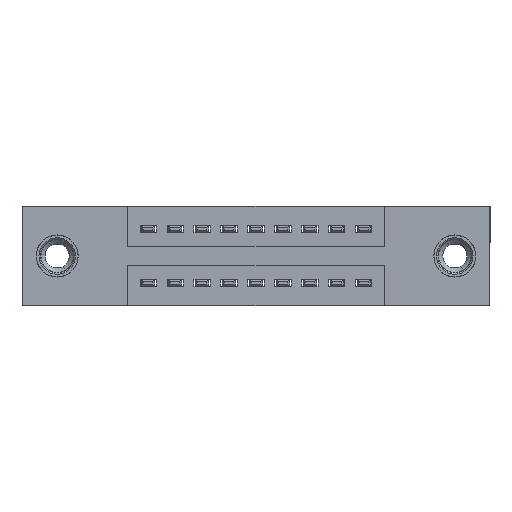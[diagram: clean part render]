
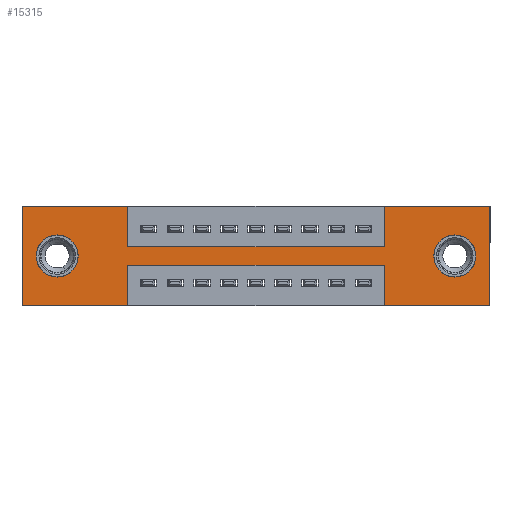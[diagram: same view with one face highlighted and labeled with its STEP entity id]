
A CAD part, front view. The second image highlights one B-rep face of the part: STEP entity #15315.
In plain terms, the highlighted planar face has unit normal (0, -1, 0).
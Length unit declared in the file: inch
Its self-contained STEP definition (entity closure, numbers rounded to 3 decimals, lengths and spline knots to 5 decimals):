
#8 = VECTOR ( 'NONE', #11460, 39.37008 ) ;
#34 = FACE_BOUND ( 'NONE', #10789, .T. ) ;
#126 = CARTESIAN_POINT ( 'NONE',  ( 1.735, 0., -0.37 ) ) ;
#457 = VECTOR ( 'NONE', #1147, 39.37008 ) ;
#826 = CARTESIAN_POINT ( 'NONE',  ( 0.3925, 0., -0.37 ) ) ;
#936 = EDGE_CURVE ( 'NONE', #4161, #10772, #6106, .T. ) ;
#960 = CARTESIAN_POINT ( 'NONE',  ( 0.3925, 0., -0.15 ) ) ;
#1044 = ORIENTED_EDGE ( 'NONE', *, *, #4124, .F. ) ;
#1058 = VERTEX_POINT ( 'NONE', #1745 ) ;
#1147 = DIRECTION ( 'NONE',  ( 0., 0., -1. ) ) ;
#1165 = VERTEX_POINT ( 'NONE', #13339 ) ;
#1525 = CARTESIAN_POINT ( 'NONE',  ( 1.3425, 0., -0.15 ) ) ;
#1726 = VERTEX_POINT ( 'NONE', #2526 ) ;
#1735 = CARTESIAN_POINT ( 'NONE',  ( 1.735, 0., 0. ) ) ;
#1745 = CARTESIAN_POINT ( 'NONE',  ( 0.13, 0., -0.263 ) ) ;
#1762 = AXIS2_PLACEMENT_3D ( 'NONE', #4137, #12771, #5459 ) ;
#1805 = AXIS2_PLACEMENT_3D ( 'NONE', #14011, #6840, #15204 ) ;
#1809 = AXIS2_PLACEMENT_3D ( 'NONE', #8352, #13079, #5833 ) ;
#1891 = CARTESIAN_POINT ( 'NONE',  ( 1.605, 0., -0.185 ) ) ;
#1919 = ORIENTED_EDGE ( 'NONE', *, *, #4104, .F. ) ;
#1977 = CARTESIAN_POINT ( 'NONE',  ( 1.3425, 0., -0.22 ) ) ;
#2094 = ORIENTED_EDGE ( 'NONE', *, *, #14705, .F. ) ;
#2177 = LINE ( 'NONE', #9393, #14913 ) ;
#2216 = LINE ( 'NONE', #7246, #14951 ) ;
#2290 = EDGE_CURVE ( 'NONE', #14207, #11654, #2216, .T. ) ;
#2526 = CARTESIAN_POINT ( 'NONE',  ( 1.3425, 0., 0. ) ) ;
#2630 = CARTESIAN_POINT ( 'NONE',  ( 0.3925, 0., -0.37 ) ) ;
#2646 = ORIENTED_EDGE ( 'NONE', *, *, #936, .F. ) ;
#2746 = FACE_BOUND ( 'NONE', #7208, .T. ) ;
#3183 = DIRECTION ( 'NONE',  ( 0., 0., -1. ) ) ;
#3472 = VERTEX_POINT ( 'NONE', #13127 ) ;
#3543 = ORIENTED_EDGE ( 'NONE', *, *, #13619, .T. ) ;
#3743 = AXIS2_PLACEMENT_3D ( 'NONE', #1891, #10708, #3183 ) ;
#3764 = VECTOR ( 'NONE', #7414, 39.37008 ) ;
#3813 = DIRECTION ( 'NONE',  ( -1., 0., 0. ) ) ;
#4104 = EDGE_CURVE ( 'NONE', #5270, #13709, #4605, .T. ) ;
#4124 = EDGE_CURVE ( 'NONE', #13709, #6918, #4186, .T. ) ;
#4137 = CARTESIAN_POINT ( 'NONE',  ( 1.605, 0., -0.185 ) ) ;
#4161 = VERTEX_POINT ( 'NONE', #13114 ) ;
#4171 = LINE ( 'NONE', #15673, #3764 ) ;
#4186 = LINE ( 'NONE', #14251, #7646 ) ;
#4452 = VERTEX_POINT ( 'NONE', #126 ) ;
#4508 = PLANE ( 'NONE',  #1809 ) ;
#4605 = LINE ( 'NONE', #11854, #13956 ) ;
#4683 = CARTESIAN_POINT ( 'NONE',  ( 0., 0., 0. ) ) ;
#4689 = EDGE_CURVE ( 'NONE', #11654, #5270, #4171, .T. ) ;
#4876 = CARTESIAN_POINT ( 'NONE',  ( 0.3925, 0., -0.22 ) ) ;
#4964 = EDGE_CURVE ( 'NONE', #3472, #14207, #7014, .T. ) ;
#4968 = CIRCLE ( 'NONE', #1762, 0.078 ) ;
#5057 = EDGE_CURVE ( 'NONE', #10867, #1058, #12298, .T. ) ;
#5081 = DIRECTION ( 'NONE',  ( 0., 1., 0. ) ) ;
#5207 = EDGE_CURVE ( 'NONE', #11205, #1726, #7616, .T. ) ;
#5270 = VERTEX_POINT ( 'NONE', #4683 ) ;
#5459 = DIRECTION ( 'NONE',  ( 0., 0., -1. ) ) ;
#5679 = DIRECTION ( 'NONE',  ( 1., 0., 0. ) ) ;
#5729 = CARTESIAN_POINT ( 'NONE',  ( 0.3925, 0., -0.15 ) ) ;
#5833 = DIRECTION ( 'NONE',  ( 0., 0., -1. ) ) ;
#5882 = CARTESIAN_POINT ( 'NONE',  ( 1.3425, 0., 0. ) ) ;
#5897 = LINE ( 'NONE', #4876, #12011 ) ;
#5986 = EDGE_CURVE ( 'NONE', #6918, #11205, #12764, .T. ) ;
#6022 = LINE ( 'NONE', #6444, #14882 ) ;
#6106 = LINE ( 'NONE', #12566, #12930 ) ;
#6213 = ORIENTED_EDGE ( 'NONE', *, *, #15624, .F. ) ;
#6444 = CARTESIAN_POINT ( 'NONE',  ( 0., 0., -0.37 ) ) ;
#6611 = EDGE_CURVE ( 'NONE', #10772, #3472, #5897, .T. ) ;
#6775 = ORIENTED_EDGE ( 'NONE', *, *, #2290, .F. ) ;
#6840 = DIRECTION ( 'NONE',  ( 0., 1., 0. ) ) ;
#6918 = VERTEX_POINT ( 'NONE', #5729 ) ;
#6990 = DIRECTION ( 'NONE',  ( 1., 0., 0. ) ) ;
#7014 = LINE ( 'NONE', #2630, #8 ) ;
#7073 = EDGE_CURVE ( 'NONE', #1058, #10867, #14374, .T. ) ;
#7094 = DIRECTION ( 'NONE',  ( 0., 0., -1. ) ) ;
#7132 = ORIENTED_EDGE ( 'NONE', *, *, #5057, .T. ) ;
#7208 = EDGE_LOOP ( 'NONE', ( #3543, #15861 ) ) ;
#7246 = CARTESIAN_POINT ( 'NONE',  ( 0., 0., -0.37 ) ) ;
#7414 = DIRECTION ( 'NONE',  ( 0., 0., 1. ) ) ;
#7616 = LINE ( 'NONE', #5882, #10794 ) ;
#7646 = VECTOR ( 'NONE', #7094, 39.37008 ) ;
#7765 = VERTEX_POINT ( 'NONE', #8893 ) ;
#7897 = CARTESIAN_POINT ( 'NONE',  ( 0., 0., -0.37 ) ) ;
#8352 = CARTESIAN_POINT ( 'NONE',  ( 0., 0., -0.37 ) ) ;
#8463 = ORIENTED_EDGE ( 'NONE', *, *, #7073, .T. ) ;
#8473 = ORIENTED_EDGE ( 'NONE', *, *, #5986, .F. ) ;
#8501 = CARTESIAN_POINT ( 'NONE',  ( 0.3925, 0., 0. ) ) ;
#8893 = CARTESIAN_POINT ( 'NONE',  ( 1.605, 0., -0.107 ) ) ;
#9007 = CIRCLE ( 'NONE', #3743, 0.078 ) ;
#9393 = CARTESIAN_POINT ( 'NONE',  ( 0., 0., 0. ) ) ;
#9606 = VECTOR ( 'NONE', #13431, 39.37008 ) ;
#9949 = EDGE_CURVE ( 'NONE', #11763, #4452, #10622, .T. ) ;
#10062 = ORIENTED_EDGE ( 'NONE', *, *, #6611, .F. ) ;
#10617 = EDGE_CURVE ( 'NONE', #1165, #7765, #4968, .T. ) ;
#10622 = LINE ( 'NONE', #15905, #457 ) ;
#10664 = ORIENTED_EDGE ( 'NONE', *, *, #5207, .F. ) ;
#10708 = DIRECTION ( 'NONE',  ( 0., 1., 0. ) ) ;
#10772 = VERTEX_POINT ( 'NONE', #1977 ) ;
#10789 = EDGE_LOOP ( 'NONE', ( #7132, #8463 ) ) ;
#10794 = VECTOR ( 'NONE', #11974, 39.37008 ) ;
#10867 = VERTEX_POINT ( 'NONE', #15685 ) ;
#11205 = VERTEX_POINT ( 'NONE', #1525 ) ;
#11275 = ORIENTED_EDGE ( 'NONE', *, *, #4689, .F. ) ;
#11460 = DIRECTION ( 'NONE',  ( 0., 0., -1. ) ) ;
#11654 = VERTEX_POINT ( 'NONE', #7897 ) ;
#11763 = VERTEX_POINT ( 'NONE', #1735 ) ;
#11854 = CARTESIAN_POINT ( 'NONE',  ( 0., 0., 0. ) ) ;
#11974 = DIRECTION ( 'NONE',  ( 0., 0., 1. ) ) ;
#12011 = VECTOR ( 'NONE', #15775, 39.37008 ) ;
#12298 = CIRCLE ( 'NONE', #1805, 0.078 ) ;
#12433 = CARTESIAN_POINT ( 'NONE',  ( 0.13, 0., -0.185 ) ) ;
#12566 = CARTESIAN_POINT ( 'NONE',  ( 1.3425, 0., -0.37 ) ) ;
#12677 = FACE_OUTER_BOUND ( 'NONE', #14859, .T. ) ;
#12764 = LINE ( 'NONE', #960, #9606 ) ;
#12771 = DIRECTION ( 'NONE',  ( 0., 1., 0. ) ) ;
#12884 = DIRECTION ( 'NONE',  ( -1., 0., 0. ) ) ;
#12930 = VECTOR ( 'NONE', #13647, 39.37008 ) ;
#13079 = DIRECTION ( 'NONE',  ( 0., -1., 0. ) ) ;
#13114 = CARTESIAN_POINT ( 'NONE',  ( 1.3425, 0., -0.37 ) ) ;
#13127 = CARTESIAN_POINT ( 'NONE',  ( 0.3925, 0., -0.22 ) ) ;
#13339 = CARTESIAN_POINT ( 'NONE',  ( 1.605, 0., -0.263 ) ) ;
#13431 = DIRECTION ( 'NONE',  ( 1., 0., 0. ) ) ;
#13518 = ORIENTED_EDGE ( 'NONE', *, *, #4964, .F. ) ;
#13599 = DIRECTION ( 'NONE',  ( 0., 0., 1. ) ) ;
#13619 = EDGE_CURVE ( 'NONE', #7765, #1165, #9007, .T. ) ;
#13647 = DIRECTION ( 'NONE',  ( 0., 0., 1. ) ) ;
#13709 = VERTEX_POINT ( 'NONE', #8501 ) ;
#13956 = VECTOR ( 'NONE', #6990, 39.37008 ) ;
#14011 = CARTESIAN_POINT ( 'NONE',  ( 0.13, 0., -0.185 ) ) ;
#14207 = VERTEX_POINT ( 'NONE', #826 ) ;
#14251 = CARTESIAN_POINT ( 'NONE',  ( 0.3925, 0., 0. ) ) ;
#14374 = CIRCLE ( 'NONE', #15145, 0.078 ) ;
#14705 = EDGE_CURVE ( 'NONE', #1726, #11763, #2177, .T. ) ;
#14818 = ORIENTED_EDGE ( 'NONE', *, *, #9949, .F. ) ;
#14859 = EDGE_LOOP ( 'NONE', ( #13518, #10062, #2646, #6213, #14818, #2094, #10664, #8473, #1044, #1919, #11275, #6775 ) ) ;
#14882 = VECTOR ( 'NONE', #3813, 39.37008 ) ;
#14913 = VECTOR ( 'NONE', #5679, 39.37008 ) ;
#14951 = VECTOR ( 'NONE', #12884, 39.37008 ) ;
#15145 = AXIS2_PLACEMENT_3D ( 'NONE', #12433, #5081, #13599 ) ;
#15204 = DIRECTION ( 'NONE',  ( 0., 0., 1. ) ) ;
#15315 = ADVANCED_FACE ( 'NONE', ( #2746, #34, #12677 ), #4508, .T. ) ;
#15624 = EDGE_CURVE ( 'NONE', #4452, #4161, #6022, .T. ) ;
#15673 = CARTESIAN_POINT ( 'NONE',  ( 0., 0., 0. ) ) ;
#15685 = CARTESIAN_POINT ( 'NONE',  ( 0.13, 0., -0.107 ) ) ;
#15775 = DIRECTION ( 'NONE',  ( -1., 0., 0. ) ) ;
#15861 = ORIENTED_EDGE ( 'NONE', *, *, #10617, .T. ) ;
#15905 = CARTESIAN_POINT ( 'NONE',  ( 1.735, 0., 0. ) ) ;
